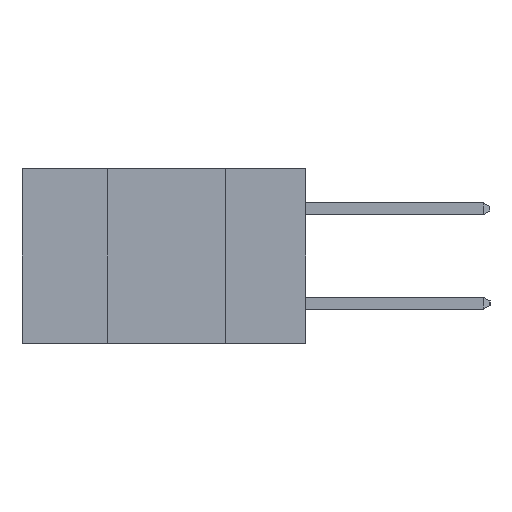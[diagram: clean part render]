
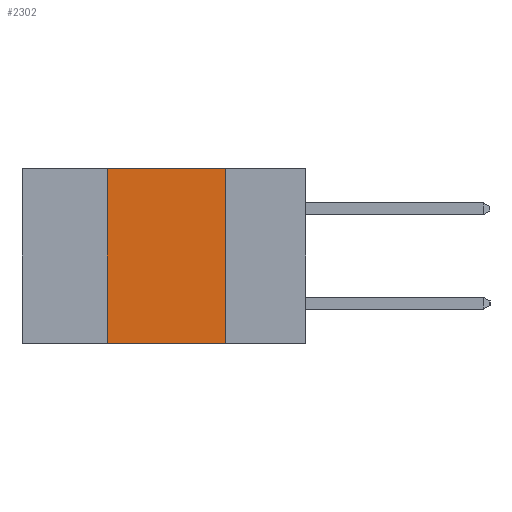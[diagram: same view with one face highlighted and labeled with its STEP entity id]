
A CAD part, left-side view. The second image highlights one B-rep face of the part: STEP entity #2302.
In plain terms, the highlighted planar face has unit normal (-1, 0, 0).
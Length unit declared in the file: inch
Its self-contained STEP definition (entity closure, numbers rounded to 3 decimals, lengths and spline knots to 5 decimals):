
#481 = VERTEX_POINT ( 'NONE', #2295 ) ;
#1560 = EDGE_CURVE ( 'NONE', #481, #9723, #8289, .T. ) ;
#2295 = CARTESIAN_POINT ( 'NONE',  ( 0., 0.42, -0.37 ) ) ;
#2302 = ADVANCED_FACE ( 'NONE', ( #9794 ), #10049, .F. ) ;
#2735 = VECTOR ( 'NONE', #7599, 39.37008 ) ;
#3572 = ORIENTED_EDGE ( 'NONE', *, *, #6905, .T. ) ;
#3652 = CARTESIAN_POINT ( 'NONE',  ( 0., 0.17, -0.37 ) ) ;
#3957 = DIRECTION ( 'NONE',  ( 0., 0., 1. ) ) ;
#4048 = ORIENTED_EDGE ( 'NONE', *, *, #10721, .F. ) ;
#4635 = VECTOR ( 'NONE', #9583, 39.37008 ) ;
#4964 = LINE ( 'NONE', #10052, #2735 ) ;
#5018 = DIRECTION ( 'NONE',  ( 0., -1., 0. ) ) ;
#5057 = VECTOR ( 'NONE', #5018, 39.37008 ) ;
#5759 = VECTOR ( 'NONE', #3957, 39.37008 ) ;
#5847 = CARTESIAN_POINT ( 'NONE',  ( 0., 0.42, 0. ) ) ;
#6905 = EDGE_CURVE ( 'NONE', #481, #7160, #4964, .T. ) ;
#7160 = VERTEX_POINT ( 'NONE', #3652 ) ;
#7599 = DIRECTION ( 'NONE',  ( 0., -1., 0. ) ) ;
#8289 = LINE ( 'NONE', #9376, #5759 ) ;
#8339 = CARTESIAN_POINT ( 'NONE',  ( 0., 0.17, 0. ) ) ;
#8499 = EDGE_CURVE ( 'NONE', #9723, #9692, #9518, .T. ) ;
#8778 = CARTESIAN_POINT ( 'NONE',  ( 0., 0.17, -0.37 ) ) ;
#9102 = AXIS2_PLACEMENT_3D ( 'NONE', #9809, #10024, #10164 ) ;
#9352 = LINE ( 'NONE', #8778, #4635 ) ;
#9376 = CARTESIAN_POINT ( 'NONE',  ( 0., 0.42, -0.37 ) ) ;
#9518 = LINE ( 'NONE', #10837, #5057 ) ;
#9583 = DIRECTION ( 'NONE',  ( 0., 0., -1. ) ) ;
#9692 = VERTEX_POINT ( 'NONE', #8339 ) ;
#9723 = VERTEX_POINT ( 'NONE', #5847 ) ;
#9731 = EDGE_LOOP ( 'NONE', ( #4048, #9855, #9869, #3572 ) ) ;
#9794 = FACE_OUTER_BOUND ( 'NONE', #9731, .T. ) ;
#9809 = CARTESIAN_POINT ( 'NONE',  ( 0., 0.6, 0. ) ) ;
#9855 = ORIENTED_EDGE ( 'NONE', *, *, #8499, .F. ) ;
#9869 = ORIENTED_EDGE ( 'NONE', *, *, #1560, .F. ) ;
#10024 = DIRECTION ( 'NONE',  ( 1., 0., 0. ) ) ;
#10049 = PLANE ( 'NONE',  #9102 ) ;
#10052 = CARTESIAN_POINT ( 'NONE',  ( 0., 0.6, -0.37 ) ) ;
#10164 = DIRECTION ( 'NONE',  ( 0., 0., -1. ) ) ;
#10721 = EDGE_CURVE ( 'NONE', #9692, #7160, #9352, .T. ) ;
#10837 = CARTESIAN_POINT ( 'NONE',  ( 0., 0.6, 0. ) ) ;
